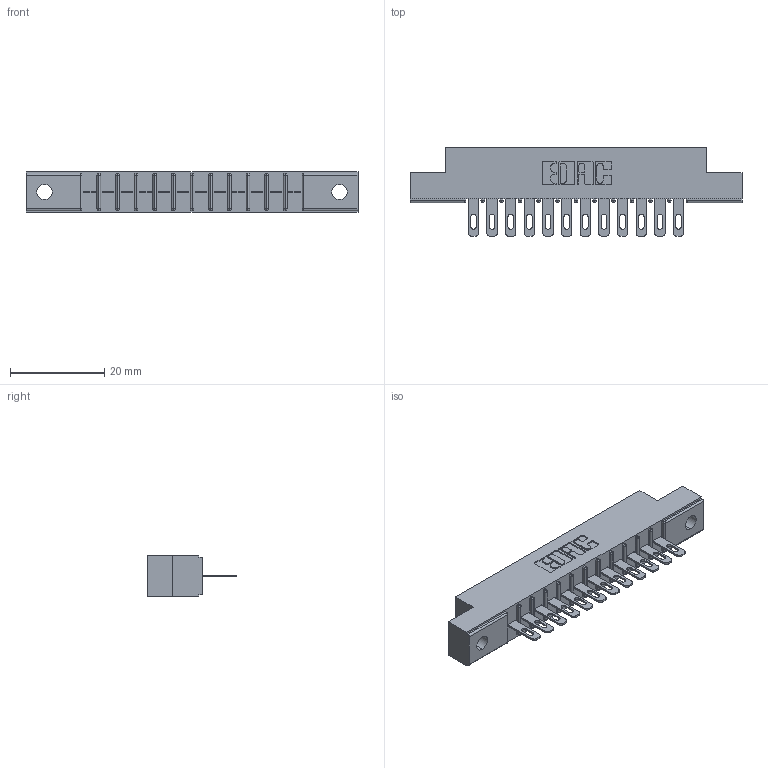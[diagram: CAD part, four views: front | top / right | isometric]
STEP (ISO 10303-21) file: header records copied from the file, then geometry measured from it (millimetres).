
FILE_DESCRIPTION (( 'STEP AP203' ), '1' );
FILE_NAME ('306-012-500-102.STEP', '2019-09-11T19:29:50', ( '' ), ( '' ), 'SwSTEP 2.0', 'SolidWorks 2016', '' );
FILE_SCHEMA (( 'CONFIG_CONTROL_DESIGN' ));
Length unit declared in the file: inch
Products named in the file (3): 306-012-500-102; 306 Part_.128 Dia; 306-290-001_100
Assembly tree (13 placements, depth 2):
  306-012-500-102
    306 Part_.128 Dia
    306-290-001_100  x12
Bounding box: 70.56 x 18.87 x 8.71 mm (x, y, z)
Volume: 4779.6 mm3; surface area: 6690.5 mm2
Topology: 13 solids, 13 shells, 1028 faces, 2896 edges, 1864 vertices
Faces by surface type: plane 668, cylinder 312, sphere 48
Entity records: 15243 total; most frequent: CARTESIAN_POINT 2555, ORIENTED_EDGE 2528, DIRECTION 2524, EDGE_CURVE 1264, LINE 970, VECTOR 970, VERTEX_POINT 808, AXIS2_PLACEMENT_3D 777
